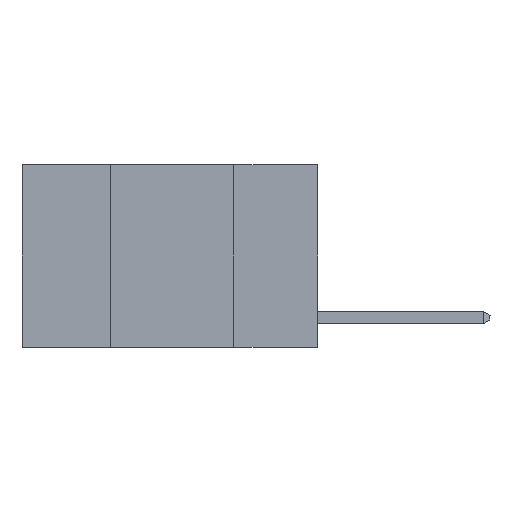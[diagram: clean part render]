
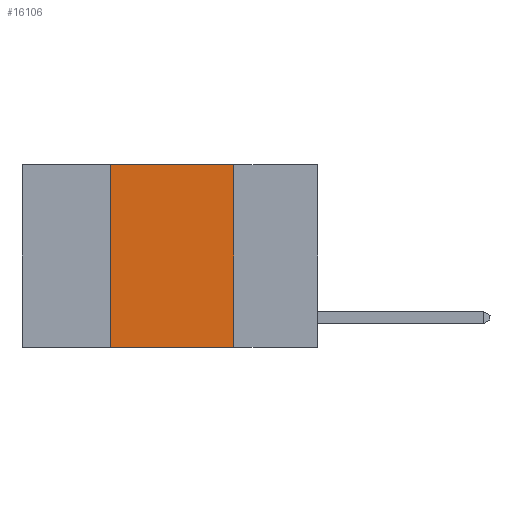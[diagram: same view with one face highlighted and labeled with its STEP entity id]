
A CAD part, left-side view. The second image highlights one B-rep face of the part: STEP entity #16106.
In plain terms, the highlighted planar face has unit normal (-1, 0, 0).
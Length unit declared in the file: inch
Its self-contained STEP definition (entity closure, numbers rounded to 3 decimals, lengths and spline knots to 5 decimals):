
#21 = VERTEX_POINT ( 'NONE', #10130 ) ;
#579 = LINE ( 'NONE', #14465, #3331 ) ;
#633 = FACE_OUTER_BOUND ( 'NONE', #9424, .T. ) ;
#943 = ORIENTED_EDGE ( 'NONE', *, *, #11057, .F. ) ;
#1251 = DIRECTION ( 'NONE',  ( 1., 0., 0. ) ) ;
#2469 = CARTESIAN_POINT ( 'NONE',  ( 0., 0.42, -0.37 ) ) ;
#2534 = DIRECTION ( 'NONE',  ( 0., 0., -1. ) ) ;
#2770 = DIRECTION ( 'NONE',  ( 0., -1., 0. ) ) ;
#3238 = VECTOR ( 'NONE', #9349, 39.37008 ) ;
#3331 = VECTOR ( 'NONE', #9337, 39.37008 ) ;
#4424 = CARTESIAN_POINT ( 'NONE',  ( 0., 0.17, -0.37 ) ) ;
#5121 = EDGE_CURVE ( 'NONE', #21, #8892, #579, .T. ) ;
#5634 = VECTOR ( 'NONE', #15175, 39.37008 ) ;
#6468 = CARTESIAN_POINT ( 'NONE',  ( 0., 0.42, 0. ) ) ;
#6721 = ORIENTED_EDGE ( 'NONE', *, *, #8631, .T. ) ;
#7296 = LINE ( 'NONE', #15654, #10287 ) ;
#8631 = EDGE_CURVE ( 'NONE', #15508, #8892, #7296, .T. ) ;
#8892 = VERTEX_POINT ( 'NONE', #4424 ) ;
#9337 = DIRECTION ( 'NONE',  ( 0., 0., -1. ) ) ;
#9349 = DIRECTION ( 'NONE',  ( 0., -1., 0. ) ) ;
#9424 = EDGE_LOOP ( 'NONE', ( #12775, #9504, #943, #6721 ) ) ;
#9504 = ORIENTED_EDGE ( 'NONE', *, *, #11216, .F. ) ;
#10130 = CARTESIAN_POINT ( 'NONE',  ( 0., 0.17, 0. ) ) ;
#10232 = CARTESIAN_POINT ( 'NONE',  ( 0., 0.6, 0. ) ) ;
#10287 = VECTOR ( 'NONE', #2770, 39.37008 ) ;
#10418 = LINE ( 'NONE', #11383, #5634 ) ;
#10649 = CARTESIAN_POINT ( 'NONE',  ( 0., 0.6, 0. ) ) ;
#11057 = EDGE_CURVE ( 'NONE', #15508, #11583, #10418, .T. ) ;
#11216 = EDGE_CURVE ( 'NONE', #11583, #21, #11618, .T. ) ;
#11383 = CARTESIAN_POINT ( 'NONE',  ( 0., 0.42, 0. ) ) ;
#11396 = PLANE ( 'NONE',  #16382 ) ;
#11583 = VERTEX_POINT ( 'NONE', #6468 ) ;
#11618 = LINE ( 'NONE', #10649, #3238 ) ;
#12775 = ORIENTED_EDGE ( 'NONE', *, *, #5121, .F. ) ;
#14465 = CARTESIAN_POINT ( 'NONE',  ( 0., 0.17, 0. ) ) ;
#15175 = DIRECTION ( 'NONE',  ( 0., 0., 1. ) ) ;
#15508 = VERTEX_POINT ( 'NONE', #2469 ) ;
#15654 = CARTESIAN_POINT ( 'NONE',  ( 0., 0.6, -0.37 ) ) ;
#16106 = ADVANCED_FACE ( 'NONE', ( #633 ), #11396, .F. ) ;
#16382 = AXIS2_PLACEMENT_3D ( 'NONE', #10232, #1251, #2534 ) ;
